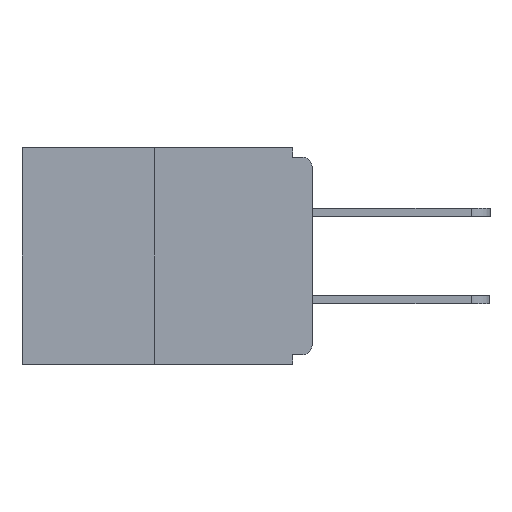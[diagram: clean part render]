
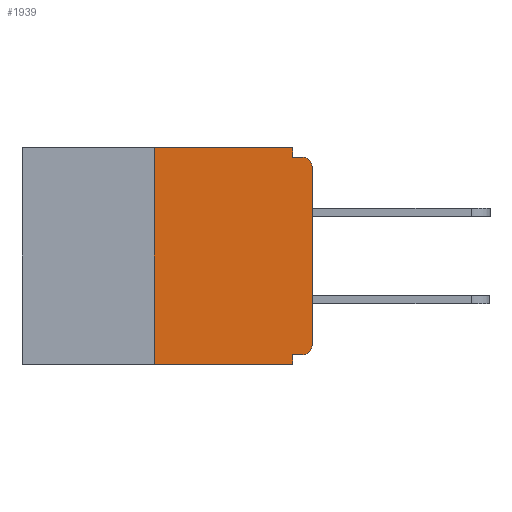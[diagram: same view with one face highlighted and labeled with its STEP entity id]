
A CAD part, left-side view. The second image highlights one B-rep face of the part: STEP entity #1939.
In plain terms, the highlighted planar face has unit normal (-1, 0, 0).
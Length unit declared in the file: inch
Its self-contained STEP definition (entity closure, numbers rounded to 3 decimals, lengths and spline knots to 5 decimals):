
#459 = AXIS2_PLACEMENT_3D ( 'NONE', #23334, #16349, #23410 ) ;
#1487 = DIRECTION ( 'NONE',  ( 0., 0., -1. ) ) ;
#1742 = VERTEX_POINT ( 'NONE', #20317 ) ;
#1939 = ADVANCED_FACE ( 'NONE', ( #21449 ), #10617, .F. ) ;
#1963 = EDGE_CURVE ( 'NONE', #21361, #18956, #12941, .T. ) ;
#2095 = DIRECTION ( 'NONE',  ( -1., 0., 0. ) ) ;
#2291 = VECTOR ( 'NONE', #14907, 39.37008 ) ;
#2755 = AXIS2_PLACEMENT_3D ( 'NONE', #3388, #10856, #1487 ) ;
#2757 = LINE ( 'NONE', #10946, #10490 ) ;
#3044 = LINE ( 'NONE', #7132, #22178 ) ;
#3340 = EDGE_CURVE ( 'NONE', #10603, #7852, #9701, .T. ) ;
#3358 = ORIENTED_EDGE ( 'NONE', *, *, #9282, .F. ) ;
#3388 = CARTESIAN_POINT ( 'NONE',  ( 0., 0.015, -0.313 ) ) ;
#3947 = CARTESIAN_POINT ( 'NONE',  ( 0., 0.031, -0.015 ) ) ;
#4177 = ORIENTED_EDGE ( 'NONE', *, *, #1963, .T. ) ;
#4408 = LINE ( 'NONE', #16068, #18723 ) ;
#4809 = VECTOR ( 'NONE', #11809, 39.37008 ) ;
#4897 = CARTESIAN_POINT ( 'NONE',  ( 0., 0., -0.328 ) ) ;
#5617 = VECTOR ( 'NONE', #15996, 39.37008 ) ;
#6002 = CIRCLE ( 'NONE', #21821, 0.015 ) ;
#6465 = EDGE_CURVE ( 'NONE', #13443, #9313, #6002, .T. ) ;
#6528 = EDGE_CURVE ( 'NONE', #18956, #13443, #12567, .T. ) ;
#6851 = DIRECTION ( 'NONE',  ( 0., -1., 0. ) ) ;
#7132 = CARTESIAN_POINT ( 'NONE',  ( 0., 0., -0.015 ) ) ;
#7195 = EDGE_CURVE ( 'NONE', #18222, #7852, #20756, .T. ) ;
#7273 = VECTOR ( 'NONE', #6851, 39.37008 ) ;
#7572 = ORIENTED_EDGE ( 'NONE', *, *, #7195, .T. ) ;
#7852 = VERTEX_POINT ( 'NONE', #20136 ) ;
#8328 = CARTESIAN_POINT ( 'NONE',  ( 0., 0., -0.03 ) ) ;
#8527 = VECTOR ( 'NONE', #8687, 39.37008 ) ;
#8636 = CARTESIAN_POINT ( 'NONE',  ( 0., 0.25, 0. ) ) ;
#8687 = DIRECTION ( 'NONE',  ( 0., -1., 0. ) ) ;
#9282 = EDGE_CURVE ( 'NONE', #18222, #17876, #4408, .T. ) ;
#9313 = VERTEX_POINT ( 'NONE', #20564 ) ;
#9589 = ORIENTED_EDGE ( 'NONE', *, *, #12964, .F. ) ;
#9701 = LINE ( 'NONE', #22707, #4809 ) ;
#10368 = CARTESIAN_POINT ( 'NONE',  ( 0., 0.46, 0. ) ) ;
#10490 = VECTOR ( 'NONE', #22094, 39.37008 ) ;
#10603 = VERTEX_POINT ( 'NONE', #11343 ) ;
#10617 = PLANE ( 'NONE',  #459 ) ;
#10856 = DIRECTION ( 'NONE',  ( -1., 0., 0. ) ) ;
#10946 = CARTESIAN_POINT ( 'NONE',  ( 0., 0.031, 0. ) ) ;
#11343 = CARTESIAN_POINT ( 'NONE',  ( 0., 0.031, -0.328 ) ) ;
#11429 = DIRECTION ( 'NONE',  ( 0., 0., -1. ) ) ;
#11809 = DIRECTION ( 'NONE',  ( 0., 0., -1. ) ) ;
#12494 = EDGE_CURVE ( 'NONE', #1742, #16981, #2757, .T. ) ;
#12567 = LINE ( 'NONE', #18775, #2291 ) ;
#12768 = LINE ( 'NONE', #4897, #5617 ) ;
#12941 = CIRCLE ( 'NONE', #2755, 0.015 ) ;
#12964 = EDGE_CURVE ( 'NONE', #21361, #10603, #12768, .T. ) ;
#13297 = CARTESIAN_POINT ( 'NONE',  ( 0., 0.25, -0.343 ) ) ;
#13443 = VERTEX_POINT ( 'NONE', #8328 ) ;
#14386 = LINE ( 'NONE', #10368, #7273 ) ;
#14907 = DIRECTION ( 'NONE',  ( 0., 0., 1. ) ) ;
#15083 = ORIENTED_EDGE ( 'NONE', *, *, #6465, .T. ) ;
#15996 = DIRECTION ( 'NONE',  ( 0., 1., 0. ) ) ;
#16052 = DIRECTION ( 'NONE',  ( 0., -1., 0. ) ) ;
#16068 = CARTESIAN_POINT ( 'NONE',  ( 0., 0.25, 0. ) ) ;
#16349 = DIRECTION ( 'NONE',  ( 1., 0., 0. ) ) ;
#16796 = CARTESIAN_POINT ( 'NONE',  ( 0., 0.015, -0.03 ) ) ;
#16981 = VERTEX_POINT ( 'NONE', #3947 ) ;
#17552 = CARTESIAN_POINT ( 'NONE',  ( 0., 0.46, -0.343 ) ) ;
#17572 = ORIENTED_EDGE ( 'NONE', *, *, #12494, .F. ) ;
#17876 = VERTEX_POINT ( 'NONE', #8636 ) ;
#18222 = VERTEX_POINT ( 'NONE', #13297 ) ;
#18444 = CARTESIAN_POINT ( 'NONE',  ( 0., 0., -0.313 ) ) ;
#18723 = VECTOR ( 'NONE', #19727, 39.37008 ) ;
#18775 = CARTESIAN_POINT ( 'NONE',  ( 0., 0., 0. ) ) ;
#18835 = ORIENTED_EDGE ( 'NONE', *, *, #3340, .F. ) ;
#18956 = VERTEX_POINT ( 'NONE', #18444 ) ;
#19727 = DIRECTION ( 'NONE',  ( 0., 0., 1. ) ) ;
#20128 = ORIENTED_EDGE ( 'NONE', *, *, #22829, .F. ) ;
#20136 = CARTESIAN_POINT ( 'NONE',  ( 0., 0.031, -0.343 ) ) ;
#20317 = CARTESIAN_POINT ( 'NONE',  ( 0., 0.031, 0. ) ) ;
#20564 = CARTESIAN_POINT ( 'NONE',  ( 0., 0.015, -0.015 ) ) ;
#20756 = LINE ( 'NONE', #17552, #8527 ) ;
#20793 = CARTESIAN_POINT ( 'NONE',  ( 0., 0.015, -0.328 ) ) ;
#21132 = EDGE_CURVE ( 'NONE', #16981, #9313, #3044, .T. ) ;
#21318 = ORIENTED_EDGE ( 'NONE', *, *, #6528, .T. ) ;
#21338 = EDGE_LOOP ( 'NONE', ( #20128, #3358, #7572, #18835, #9589, #4177, #21318, #15083, #23378, #17572 ) ) ;
#21361 = VERTEX_POINT ( 'NONE', #20793 ) ;
#21449 = FACE_OUTER_BOUND ( 'NONE', #21338, .T. ) ;
#21821 = AXIS2_PLACEMENT_3D ( 'NONE', #16796, #2095, #11429 ) ;
#22094 = DIRECTION ( 'NONE',  ( 0., 0., -1. ) ) ;
#22178 = VECTOR ( 'NONE', #16052, 39.37008 ) ;
#22707 = CARTESIAN_POINT ( 'NONE',  ( 0., 0.031, -0.343 ) ) ;
#22829 = EDGE_CURVE ( 'NONE', #17876, #1742, #14386, .T. ) ;
#23334 = CARTESIAN_POINT ( 'NONE',  ( 0., 0.46, 0. ) ) ;
#23378 = ORIENTED_EDGE ( 'NONE', *, *, #21132, .F. ) ;
#23410 = DIRECTION ( 'NONE',  ( 0., 0., -1. ) ) ;
